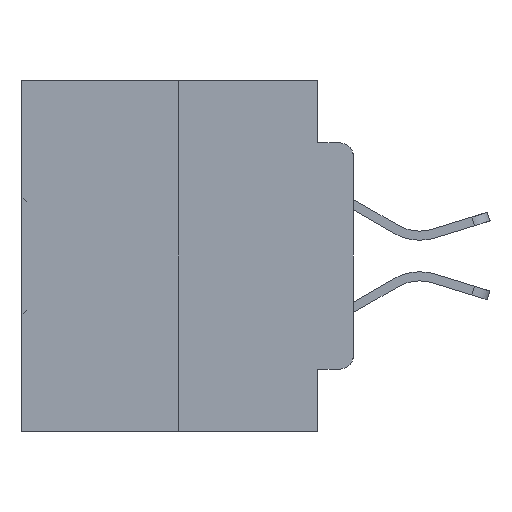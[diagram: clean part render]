
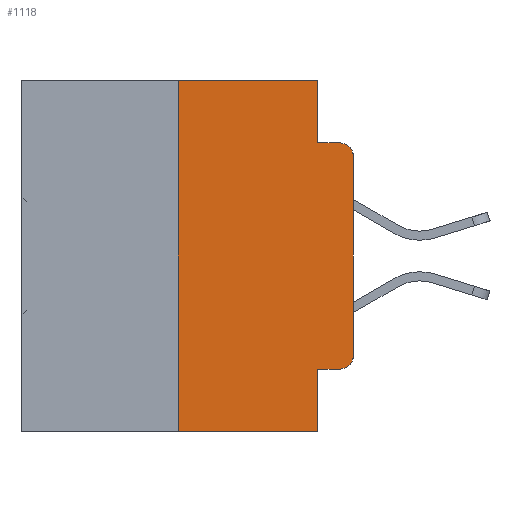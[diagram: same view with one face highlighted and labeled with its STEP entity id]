
A CAD part, left-side view. The second image highlights one B-rep face of the part: STEP entity #1118.
In plain terms, the highlighted planar face has unit normal (-1, 0, 0).
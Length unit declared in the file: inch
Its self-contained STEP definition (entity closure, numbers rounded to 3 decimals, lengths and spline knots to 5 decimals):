
#284 = AXIS2_PLACEMENT_3D ( 'NONE', #30633, #30602, #30555 ) ;
#555 = ORIENTED_EDGE ( 'NONE', *, *, #4277, .T. ) ;
#834 = VECTOR ( 'NONE', #13052, 39.37008 ) ;
#1118 = ADVANCED_FACE ( 'NONE', ( #17750 ), #11007, .F. ) ;
#1678 = ORIENTED_EDGE ( 'NONE', *, *, #12318, .F. ) ;
#1986 = AXIS2_PLACEMENT_3D ( 'NONE', #12021, #12133, #19512 ) ;
#2195 = VECTOR ( 'NONE', #28732, 39.37008 ) ;
#2359 = EDGE_CURVE ( 'NONE', #17114, #15195, #20863, .T. ) ;
#3050 = VECTOR ( 'NONE', #28527, 39.37008 ) ;
#3251 = CARTESIAN_POINT ( 'NONE',  ( 0., 0., -0.1085 ) ) ;
#3641 = EDGE_CURVE ( 'NONE', #6440, #22870, #27087, .T. ) ;
#3923 = CARTESIAN_POINT ( 'NONE',  ( 0., 0.25, -0.5 ) ) ;
#3950 = CARTESIAN_POINT ( 'NONE',  ( 0., 0.051, 0. ) ) ;
#4277 = EDGE_CURVE ( 'NONE', #21467, #6440, #8564, .T. ) ;
#4284 = CARTESIAN_POINT ( 'NONE',  ( 0., 0.051, -0.4115 ) ) ;
#5370 = CARTESIAN_POINT ( 'NONE',  ( 0., 0.051, -0.0885 ) ) ;
#5666 = LINE ( 'NONE', #3950, #19420 ) ;
#5874 = CARTESIAN_POINT ( 'NONE',  ( 0., 0.051, -0.5 ) ) ;
#6094 = DIRECTION ( 'NONE',  ( 0., 0., -1. ) ) ;
#6316 = DIRECTION ( 'NONE',  ( -1., 0., 0. ) ) ;
#6440 = VERTEX_POINT ( 'NONE', #3251 ) ;
#6604 = DIRECTION ( 'NONE',  ( 0., 0., -1. ) ) ;
#8539 = CARTESIAN_POINT ( 'NONE',  ( 0., 0.25, 0. ) ) ;
#8564 = LINE ( 'NONE', #22561, #28193 ) ;
#8691 = EDGE_CURVE ( 'NONE', #9443, #21467, #13426, .T. ) ;
#8912 = LINE ( 'NONE', #27148, #30116 ) ;
#9185 = DIRECTION ( 'NONE',  ( 0., 0., 1. ) ) ;
#9443 = VERTEX_POINT ( 'NONE', #9888 ) ;
#9888 = CARTESIAN_POINT ( 'NONE',  ( 0., 0.02, -0.4115 ) ) ;
#9957 = EDGE_CURVE ( 'NONE', #22189, #23710, #8912, .T. ) ;
#10311 = ORIENTED_EDGE ( 'NONE', *, *, #9957, .F. ) ;
#10386 = CARTESIAN_POINT ( 'NONE',  ( 0., 0.02, -0.0885 ) ) ;
#10461 = CARTESIAN_POINT ( 'NONE',  ( 0., 0.473, 0. ) ) ;
#11007 = PLANE ( 'NONE',  #1986 ) ;
#11526 = LINE ( 'NONE', #15828, #3050 ) ;
#11718 = DIRECTION ( 'NONE',  ( 0., -1., 0. ) ) ;
#12021 = CARTESIAN_POINT ( 'NONE',  ( 0., 0.473, 0. ) ) ;
#12058 = ORIENTED_EDGE ( 'NONE', *, *, #22644, .T. ) ;
#12133 = DIRECTION ( 'NONE',  ( 1., 0., 0. ) ) ;
#12318 = EDGE_CURVE ( 'NONE', #26711, #22870, #11526, .T. ) ;
#13052 = DIRECTION ( 'NONE',  ( 0., -1., 0. ) ) ;
#13375 = CARTESIAN_POINT ( 'NONE',  ( 0., 0., -0.3915 ) ) ;
#13426 = CIRCLE ( 'NONE', #17318, 0.02 ) ;
#13427 = CARTESIAN_POINT ( 'NONE',  ( 0., 0.473, -0.5 ) ) ;
#13637 = ORIENTED_EDGE ( 'NONE', *, *, #8691, .T. ) ;
#14045 = ORIENTED_EDGE ( 'NONE', *, *, #3641, .T. ) ;
#14732 = ORIENTED_EDGE ( 'NONE', *, *, #2359, .F. ) ;
#14948 = CARTESIAN_POINT ( 'NONE',  ( 0., 0.051, 0. ) ) ;
#15195 = VERTEX_POINT ( 'NONE', #5874 ) ;
#15828 = CARTESIAN_POINT ( 'NONE',  ( 0., 0.051, -0.0885 ) ) ;
#16502 = ORIENTED_EDGE ( 'NONE', *, *, #31584, .T. ) ;
#16894 = ORIENTED_EDGE ( 'NONE', *, *, #31370, .F. ) ;
#16983 = CARTESIAN_POINT ( 'NONE',  ( 0., 0.051, -0.4115 ) ) ;
#17114 = VERTEX_POINT ( 'NONE', #4284 ) ;
#17318 = AXIS2_PLACEMENT_3D ( 'NONE', #21763, #6316, #24351 ) ;
#17750 = FACE_OUTER_BOUND ( 'NONE', #27414, .T. ) ;
#19420 = VECTOR ( 'NONE', #6604, 39.37008 ) ;
#19512 = DIRECTION ( 'NONE',  ( 0., 0., -1. ) ) ;
#20863 = LINE ( 'NONE', #21886, #26862 ) ;
#21467 = VERTEX_POINT ( 'NONE', #13375 ) ;
#21485 = LINE ( 'NONE', #10461, #834 ) ;
#21525 = VECTOR ( 'NONE', #11718, 39.37008 ) ;
#21763 = CARTESIAN_POINT ( 'NONE',  ( 0., 0.02, -0.3915 ) ) ;
#21849 = LINE ( 'NONE', #16983, #21525 ) ;
#21886 = CARTESIAN_POINT ( 'NONE',  ( 0., 0.051, 0. ) ) ;
#22189 = VERTEX_POINT ( 'NONE', #3923 ) ;
#22349 = ORIENTED_EDGE ( 'NONE', *, *, #32826, .F. ) ;
#22561 = CARTESIAN_POINT ( 'NONE',  ( 0., 0., 0. ) ) ;
#22644 = EDGE_CURVE ( 'NONE', #22189, #15195, #22827, .T. ) ;
#22688 = DIRECTION ( 'NONE',  ( 0., 0., 1. ) ) ;
#22827 = LINE ( 'NONE', #13427, #2195 ) ;
#22870 = VERTEX_POINT ( 'NONE', #10386 ) ;
#23710 = VERTEX_POINT ( 'NONE', #8539 ) ;
#24351 = DIRECTION ( 'NONE',  ( 0., 0., -1. ) ) ;
#26711 = VERTEX_POINT ( 'NONE', #5370 ) ;
#26862 = VECTOR ( 'NONE', #6094, 39.37008 ) ;
#27087 = CIRCLE ( 'NONE', #284, 0.02 ) ;
#27148 = CARTESIAN_POINT ( 'NONE',  ( 0., 0.25, 0. ) ) ;
#27414 = EDGE_LOOP ( 'NONE', ( #555, #14045, #1678, #22349, #16894, #10311, #12058, #14732, #16502, #13637 ) ) ;
#28193 = VECTOR ( 'NONE', #22688, 39.37008 ) ;
#28527 = DIRECTION ( 'NONE',  ( 0., -1., 0. ) ) ;
#28732 = DIRECTION ( 'NONE',  ( 0., -1., 0. ) ) ;
#29979 = VERTEX_POINT ( 'NONE', #14948 ) ;
#30116 = VECTOR ( 'NONE', #9185, 39.37008 ) ;
#30555 = DIRECTION ( 'NONE',  ( 0., 0., -1. ) ) ;
#30602 = DIRECTION ( 'NONE',  ( -1., 0., 0. ) ) ;
#30633 = CARTESIAN_POINT ( 'NONE',  ( 0., 0.02, -0.1085 ) ) ;
#31370 = EDGE_CURVE ( 'NONE', #23710, #29979, #21485, .T. ) ;
#31584 = EDGE_CURVE ( 'NONE', #17114, #9443, #21849, .T. ) ;
#32826 = EDGE_CURVE ( 'NONE', #29979, #26711, #5666, .T. ) ;
